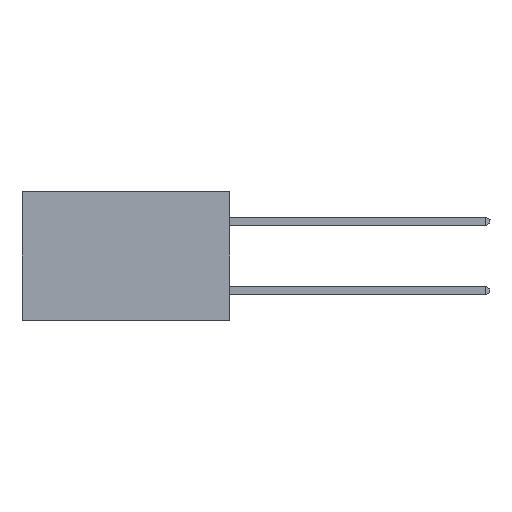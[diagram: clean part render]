
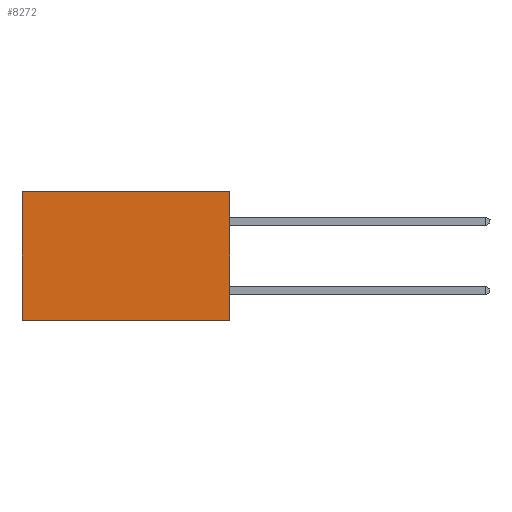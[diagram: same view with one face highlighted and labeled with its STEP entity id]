
A CAD part, left-side view. The second image highlights one B-rep face of the part: STEP entity #8272.
In plain terms, the highlighted planar face has unit normal (-1, 0, 0).
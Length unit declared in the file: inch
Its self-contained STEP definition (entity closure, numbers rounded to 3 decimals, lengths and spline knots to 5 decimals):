
#2062 = FACE_OUTER_BOUND ( 'NONE', #18249, .T. ) ;
#2364 = CARTESIAN_POINT ( 'NONE',  ( 0.298, 0.6, 0. ) ) ;
#2829 = CARTESIAN_POINT ( 'NONE',  ( 0.298, 0.6, -0.37 ) ) ;
#3057 = LINE ( 'NONE', #17832, #9738 ) ;
#3143 = CARTESIAN_POINT ( 'NONE',  ( 0.298, 0., 0. ) ) ;
#3427 = DIRECTION ( 'NONE',  ( 0., 0., -1. ) ) ;
#3858 = CARTESIAN_POINT ( 'NONE',  ( 0.298, 0., -0.37 ) ) ;
#4910 = CARTESIAN_POINT ( 'NONE',  ( 0.298, 0., 0. ) ) ;
#5160 = DIRECTION ( 'NONE',  ( 0., 0., -1. ) ) ;
#5444 = AXIS2_PLACEMENT_3D ( 'NONE', #4910, #8410, #3427 ) ;
#5477 = ORIENTED_EDGE ( 'NONE', *, *, #10305, .T. ) ;
#6099 = VERTEX_POINT ( 'NONE', #3143 ) ;
#8095 = CARTESIAN_POINT ( 'NONE',  ( 0.298, 0., -0.37 ) ) ;
#8272 = ADVANCED_FACE ( 'NONE', ( #2062 ), #10047, .F. ) ;
#8410 = DIRECTION ( 'NONE',  ( 1., 0., 0. ) ) ;
#8473 = EDGE_CURVE ( 'NONE', #6099, #13023, #3057, .T. ) ;
#8735 = ORIENTED_EDGE ( 'NONE', *, *, #19002, .F. ) ;
#9160 = VECTOR ( 'NONE', #5160, 39.37008 ) ;
#9339 = DIRECTION ( 'NONE',  ( 0., 1., 0. ) ) ;
#9738 = VECTOR ( 'NONE', #9339, 39.37008 ) ;
#10047 = PLANE ( 'NONE',  #5444 ) ;
#10305 = EDGE_CURVE ( 'NONE', #13023, #15079, #16088, .T. ) ;
#11112 = VECTOR ( 'NONE', #16667, 39.37008 ) ;
#12176 = LINE ( 'NONE', #8095, #11112 ) ;
#12565 = LINE ( 'NONE', #16080, #18695 ) ;
#13023 = VERTEX_POINT ( 'NONE', #2364 ) ;
#14291 = DIRECTION ( 'NONE',  ( 0., 0., -1. ) ) ;
#15079 = VERTEX_POINT ( 'NONE', #2829 ) ;
#15342 = CARTESIAN_POINT ( 'NONE',  ( 0.298, 0.6, 0. ) ) ;
#16080 = CARTESIAN_POINT ( 'NONE',  ( 0.298, 0., 0. ) ) ;
#16088 = LINE ( 'NONE', #15342, #9160 ) ;
#16667 = DIRECTION ( 'NONE',  ( 0., 1., 0. ) ) ;
#17301 = ORIENTED_EDGE ( 'NONE', *, *, #21918, .F. ) ;
#17832 = CARTESIAN_POINT ( 'NONE',  ( 0.298, 0., 0. ) ) ;
#17993 = ORIENTED_EDGE ( 'NONE', *, *, #8473, .T. ) ;
#18249 = EDGE_LOOP ( 'NONE', ( #5477, #17301, #8735, #17993 ) ) ;
#18695 = VECTOR ( 'NONE', #14291, 39.37008 ) ;
#19002 = EDGE_CURVE ( 'NONE', #6099, #21205, #12565, .T. ) ;
#21205 = VERTEX_POINT ( 'NONE', #3858 ) ;
#21918 = EDGE_CURVE ( 'NONE', #21205, #15079, #12176, .T. ) ;
